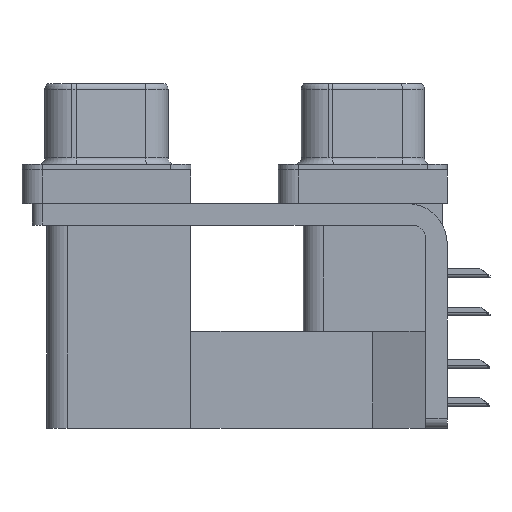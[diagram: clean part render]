
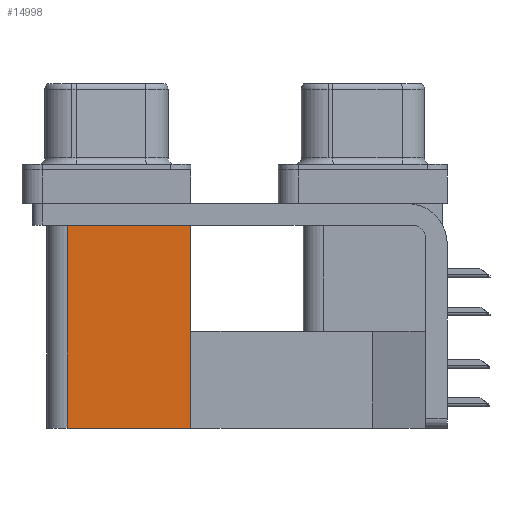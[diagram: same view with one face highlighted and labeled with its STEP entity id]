
A CAD part, left-side view. The second image highlights one B-rep face of the part: STEP entity #14998.
In plain terms, the highlighted planar face has unit normal (-1, 0, 0).
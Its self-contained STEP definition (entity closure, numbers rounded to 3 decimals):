
#427 = FACE_OUTER_BOUND ( 'NONE', #3974, .T. ) ;
#608 = CARTESIAN_POINT ( 'NONE',  ( 3.79, 12.775, -2.5 ) ) ;
#727 = VECTOR ( 'NONE', #3298, 1000. ) ;
#1206 = VECTOR ( 'NONE', #20642, 1000. ) ;
#1497 = LINE ( 'NONE', #8683, #21166 ) ;
#2370 = CARTESIAN_POINT ( 'NONE',  ( 3.79, 12.775, -2.5 ) ) ;
#3298 = DIRECTION ( 'NONE',  ( 0., 1., 0. ) ) ;
#3380 = DIRECTION ( 'NONE',  ( 0., 0., 1. ) ) ;
#3744 = ORIENTED_EDGE ( 'NONE', *, *, #10733, .F. ) ;
#3974 = EDGE_LOOP ( 'NONE', ( #18920, #3744, #4850, #4750 ) ) ;
#4750 = ORIENTED_EDGE ( 'NONE', *, *, #16107, .T. ) ;
#4850 = ORIENTED_EDGE ( 'NONE', *, *, #11497, .F. ) ;
#6896 = CARTESIAN_POINT ( 'NONE',  ( 3.79, 21.975, -19.2 ) ) ;
#7510 = PLANE ( 'NONE',  #12075 ) ;
#7624 = CARTESIAN_POINT ( 'NONE',  ( 3.79, 12.775, -19.2 ) ) ;
#8120 = VERTEX_POINT ( 'NONE', #17718 ) ;
#8683 = CARTESIAN_POINT ( 'NONE',  ( 3.79, 12.775, -19.2 ) ) ;
#10079 = VERTEX_POINT ( 'NONE', #608 ) ;
#10733 = EDGE_CURVE ( 'NONE', #8120, #19465, #23047, .T. ) ;
#11381 = DIRECTION ( 'NONE',  ( 1., 0., 0. ) ) ;
#11497 = EDGE_CURVE ( 'NONE', #11514, #8120, #12248, .T. ) ;
#11514 = VERTEX_POINT ( 'NONE', #15671 ) ;
#12075 = AXIS2_PLACEMENT_3D ( 'NONE', #7624, #11381, #14927 ) ;
#12248 = LINE ( 'NONE', #15554, #727 ) ;
#12297 = DIRECTION ( 'NONE',  ( 0., 0., 1. ) ) ;
#13428 = LINE ( 'NONE', #2370, #1206 ) ;
#13900 = CARTESIAN_POINT ( 'NONE',  ( 3.79, 21.975, -2.5 ) ) ;
#14196 = EDGE_CURVE ( 'NONE', #10079, #19465, #13428, .T. ) ;
#14927 = DIRECTION ( 'NONE',  ( 0., 0., -1. ) ) ;
#14998 = ADVANCED_FACE ( 'NONE', ( #427 ), #7510, .F. ) ;
#15554 = CARTESIAN_POINT ( 'NONE',  ( 3.79, 12.775, -19.2 ) ) ;
#15671 = CARTESIAN_POINT ( 'NONE',  ( 3.79, 12.775, -19.2 ) ) ;
#16107 = EDGE_CURVE ( 'NONE', #11514, #10079, #1497, .T. ) ;
#17718 = CARTESIAN_POINT ( 'NONE',  ( 3.79, 21.975, -19.2 ) ) ;
#18920 = ORIENTED_EDGE ( 'NONE', *, *, #14196, .T. ) ;
#19465 = VERTEX_POINT ( 'NONE', #13900 ) ;
#20642 = DIRECTION ( 'NONE',  ( 0., 1., 0. ) ) ;
#21166 = VECTOR ( 'NONE', #3380, 1000. ) ;
#22160 = VECTOR ( 'NONE', #12297, 1000. ) ;
#23047 = LINE ( 'NONE', #6896, #22160 ) ;
